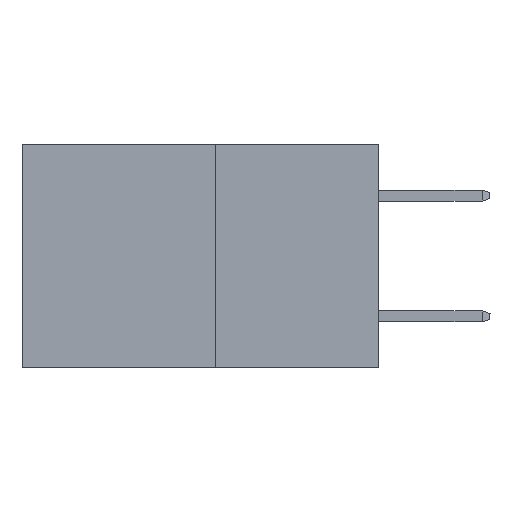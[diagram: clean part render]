
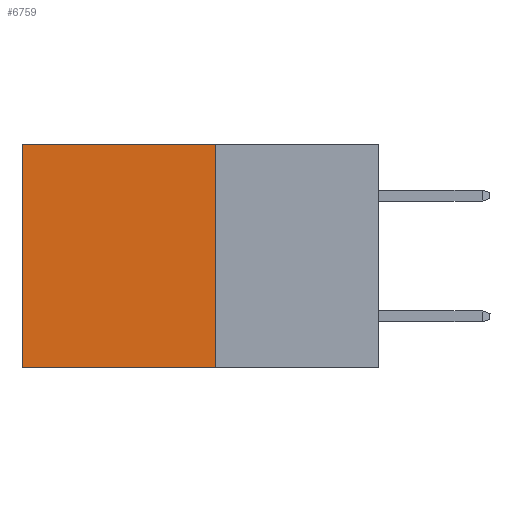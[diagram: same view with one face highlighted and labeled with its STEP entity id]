
A CAD part, left-side view. The second image highlights one B-rep face of the part: STEP entity #6759.
In plain terms, the highlighted planar face has unit normal (-1, 0, 0).
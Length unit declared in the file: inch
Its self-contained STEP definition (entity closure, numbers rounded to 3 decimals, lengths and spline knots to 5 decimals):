
#366 = DIRECTION ( 'NONE',  ( 0., 0., -1. ) ) ;
#377 = DIRECTION ( 'NONE',  ( 1., 0., 0. ) ) ;
#411 = CARTESIAN_POINT ( 'NONE',  ( 0.277, 0.27, -0.37 ) ) ;
#584 = PLANE ( 'NONE',  #7553 ) ;
#599 = CARTESIAN_POINT ( 'NONE',  ( 0.277, 0.59, 0. ) ) ;
#727 = LINE ( 'NONE', #7750, #6148 ) ;
#748 = EDGE_LOOP ( 'NONE', ( #8943, #2744, #5601, #6023 ) ) ;
#896 = VERTEX_POINT ( 'NONE', #599 ) ;
#1177 = EDGE_CURVE ( 'NONE', #8738, #1867, #3384, .T. ) ;
#1255 = DIRECTION ( 'NONE',  ( 0., 0., -1. ) ) ;
#1411 = VECTOR ( 'NONE', #1255, 39.37008 ) ;
#1867 = VERTEX_POINT ( 'NONE', #8171 ) ;
#2336 = CARTESIAN_POINT ( 'NONE',  ( 0.277, 0.27, -0.37 ) ) ;
#2698 = VERTEX_POINT ( 'NONE', #8939 ) ;
#2744 = ORIENTED_EDGE ( 'NONE', *, *, #6886, .F. ) ;
#2817 = DIRECTION ( 'NONE',  ( 0., 1., 0. ) ) ;
#3046 = CARTESIAN_POINT ( 'NONE',  ( 0.277, 0.27, 0. ) ) ;
#3384 = LINE ( 'NONE', #2336, #1411 ) ;
#4330 = VECTOR ( 'NONE', #5036, 39.37008 ) ;
#5034 = CARTESIAN_POINT ( 'NONE',  ( 0.277, 0.27, 0. ) ) ;
#5036 = DIRECTION ( 'NONE',  ( 0., 1., 0. ) ) ;
#5129 = EDGE_CURVE ( 'NONE', #896, #2698, #727, .T. ) ;
#5255 = CARTESIAN_POINT ( 'NONE',  ( 0.277, 0.27, -0.37 ) ) ;
#5601 = ORIENTED_EDGE ( 'NONE', *, *, #1177, .F. ) ;
#6023 = ORIENTED_EDGE ( 'NONE', *, *, #6574, .T. ) ;
#6148 = VECTOR ( 'NONE', #7247, 39.37008 ) ;
#6574 = EDGE_CURVE ( 'NONE', #8738, #896, #6749, .T. ) ;
#6645 = FACE_OUTER_BOUND ( 'NONE', #748, .T. ) ;
#6749 = LINE ( 'NONE', #3046, #8349 ) ;
#6759 = ADVANCED_FACE ( 'NONE', ( #6645 ), #584, .F. ) ;
#6886 = EDGE_CURVE ( 'NONE', #1867, #2698, #7578, .T. ) ;
#7247 = DIRECTION ( 'NONE',  ( 0., 0., -1. ) ) ;
#7553 = AXIS2_PLACEMENT_3D ( 'NONE', #411, #377, #366 ) ;
#7578 = LINE ( 'NONE', #5255, #4330 ) ;
#7750 = CARTESIAN_POINT ( 'NONE',  ( 0.277, 0.59, -0.37 ) ) ;
#8171 = CARTESIAN_POINT ( 'NONE',  ( 0.277, 0.27, -0.37 ) ) ;
#8349 = VECTOR ( 'NONE', #2817, 39.37008 ) ;
#8738 = VERTEX_POINT ( 'NONE', #5034 ) ;
#8939 = CARTESIAN_POINT ( 'NONE',  ( 0.277, 0.59, -0.37 ) ) ;
#8943 = ORIENTED_EDGE ( 'NONE', *, *, #5129, .T. ) ;
